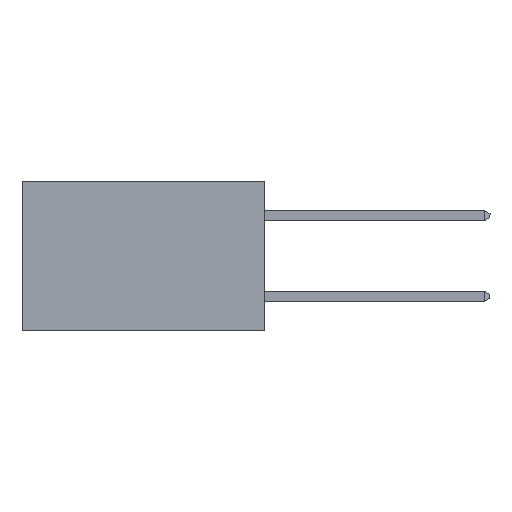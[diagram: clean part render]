
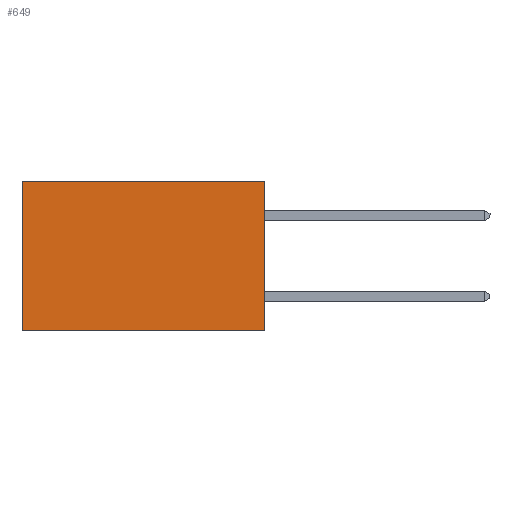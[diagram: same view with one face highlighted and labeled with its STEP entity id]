
A CAD part, left-side view. The second image highlights one B-rep face of the part: STEP entity #649.
In plain terms, the highlighted planar face has unit normal (-1, 0, 0).
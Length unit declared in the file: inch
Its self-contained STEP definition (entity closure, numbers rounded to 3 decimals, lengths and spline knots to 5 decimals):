
#100 = EDGE_LOOP ( 'NONE', ( #1345, #12224, #11460, #7445 ) ) ;
#649 = ADVANCED_FACE ( 'NONE', ( #2228 ), #10309, .F. ) ;
#678 = AXIS2_PLACEMENT_3D ( 'NONE', #11236, #11009, #10391 ) ;
#1018 = CARTESIAN_POINT ( 'NONE',  ( 0.298, 0., 0. ) ) ;
#1043 = CARTESIAN_POINT ( 'NONE',  ( 0.298, 0.6, -0.37 ) ) ;
#1345 = ORIENTED_EDGE ( 'NONE', *, *, #2286, .T. ) ;
#1772 = EDGE_CURVE ( 'NONE', #10948, #7135, #5719, .T. ) ;
#1937 = CARTESIAN_POINT ( 'NONE',  ( 0.298, 0., -0.37 ) ) ;
#2029 = LINE ( 'NONE', #9047, #4773 ) ;
#2228 = FACE_OUTER_BOUND ( 'NONE', #100, .T. ) ;
#2286 = EDGE_CURVE ( 'NONE', #7135, #3287, #9203, .T. ) ;
#2298 = DIRECTION ( 'NONE',  ( 0., 0., -1. ) ) ;
#2389 = DIRECTION ( 'NONE',  ( 0., 1., 0. ) ) ;
#2889 = CARTESIAN_POINT ( 'NONE',  ( 0.298, 0.6, 0. ) ) ;
#3287 = VERTEX_POINT ( 'NONE', #1043 ) ;
#4773 = VECTOR ( 'NONE', #2298, 39.37008 ) ;
#5059 = EDGE_CURVE ( 'NONE', #10948, #8007, #2029, .T. ) ;
#5206 = LINE ( 'NONE', #10841, #9764 ) ;
#5719 = LINE ( 'NONE', #1018, #10130 ) ;
#6449 = EDGE_CURVE ( 'NONE', #8007, #3287, #5206, .T. ) ;
#7135 = VERTEX_POINT ( 'NONE', #11380 ) ;
#7445 = ORIENTED_EDGE ( 'NONE', *, *, #1772, .T. ) ;
#8007 = VERTEX_POINT ( 'NONE', #1937 ) ;
#8786 = DIRECTION ( 'NONE',  ( 0., 0., -1. ) ) ;
#8931 = VECTOR ( 'NONE', #8786, 39.37008 ) ;
#9047 = CARTESIAN_POINT ( 'NONE',  ( 0.298, 0., 0. ) ) ;
#9203 = LINE ( 'NONE', #2889, #8931 ) ;
#9764 = VECTOR ( 'NONE', #2389, 39.37008 ) ;
#10041 = DIRECTION ( 'NONE',  ( 0., 1., 0. ) ) ;
#10130 = VECTOR ( 'NONE', #10041, 39.37008 ) ;
#10309 = PLANE ( 'NONE',  #678 ) ;
#10391 = DIRECTION ( 'NONE',  ( 0., 0., -1. ) ) ;
#10841 = CARTESIAN_POINT ( 'NONE',  ( 0.298, 0., -0.37 ) ) ;
#10945 = CARTESIAN_POINT ( 'NONE',  ( 0.298, 0., 0. ) ) ;
#10948 = VERTEX_POINT ( 'NONE', #10945 ) ;
#11009 = DIRECTION ( 'NONE',  ( 1., 0., 0. ) ) ;
#11236 = CARTESIAN_POINT ( 'NONE',  ( 0.298, 0., 0. ) ) ;
#11380 = CARTESIAN_POINT ( 'NONE',  ( 0.298, 0.6, 0. ) ) ;
#11460 = ORIENTED_EDGE ( 'NONE', *, *, #5059, .F. ) ;
#12224 = ORIENTED_EDGE ( 'NONE', *, *, #6449, .F. ) ;
